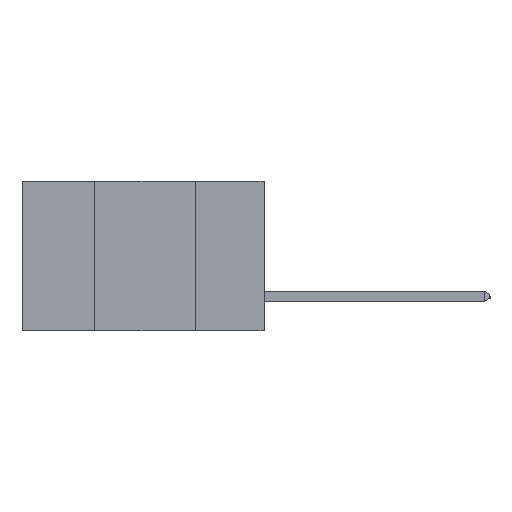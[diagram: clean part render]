
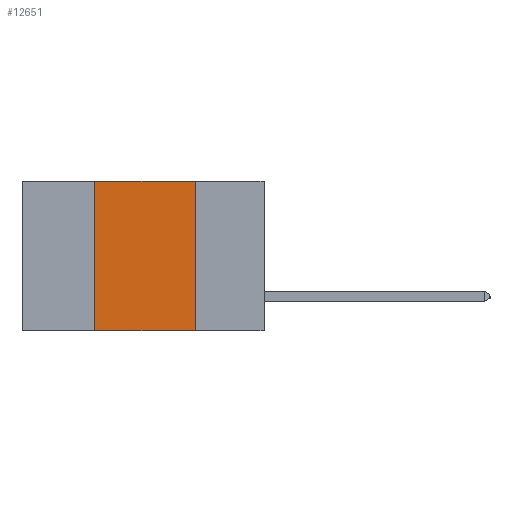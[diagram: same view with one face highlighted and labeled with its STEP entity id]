
A CAD part, left-side view. The second image highlights one B-rep face of the part: STEP entity #12651.
In plain terms, the highlighted planar face has unit normal (-1, 0, 0).
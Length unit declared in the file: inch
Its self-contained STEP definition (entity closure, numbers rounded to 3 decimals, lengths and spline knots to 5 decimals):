
#1932 = DIRECTION ( 'NONE',  ( 0., -1., 0. ) ) ;
#2040 = CARTESIAN_POINT ( 'NONE',  ( 0., 0.17, 0. ) ) ;
#2070 = EDGE_CURVE ( 'NONE', #16121, #6429, #5973, .T. ) ;
#3639 = DIRECTION ( 'NONE',  ( 0., -1., 0. ) ) ;
#4352 = EDGE_CURVE ( 'NONE', #23627, #6429, #24726, .T. ) ;
#4838 = CARTESIAN_POINT ( 'NONE',  ( 0., 0.42, -0.37 ) ) ;
#5973 = LINE ( 'NONE', #14927, #25289 ) ;
#6429 = VERTEX_POINT ( 'NONE', #12253 ) ;
#6909 = LINE ( 'NONE', #28811, #19478 ) ;
#9993 = EDGE_LOOP ( 'NONE', ( #13311, #14872, #23152, #10530 ) ) ;
#10530 = ORIENTED_EDGE ( 'NONE', *, *, #4352, .T. ) ;
#11961 = DIRECTION ( 'NONE',  ( 0., 0., -1. ) ) ;
#12033 = CARTESIAN_POINT ( 'NONE',  ( 0., 0.42, 0. ) ) ;
#12086 = VECTOR ( 'NONE', #1932, 39.37008 ) ;
#12253 = CARTESIAN_POINT ( 'NONE',  ( 0., 0.17, -0.37 ) ) ;
#12651 = ADVANCED_FACE ( 'NONE', ( #31687 ), #29521, .F. ) ;
#13311 = ORIENTED_EDGE ( 'NONE', *, *, #2070, .F. ) ;
#13995 = VERTEX_POINT ( 'NONE', #12033 ) ;
#14640 = CARTESIAN_POINT ( 'NONE',  ( 0., 0.42, 0. ) ) ;
#14872 = ORIENTED_EDGE ( 'NONE', *, *, #27193, .F. ) ;
#14927 = CARTESIAN_POINT ( 'NONE',  ( 0., 0.17, 0. ) ) ;
#16121 = VERTEX_POINT ( 'NONE', #2040 ) ;
#16141 = EDGE_CURVE ( 'NONE', #23627, #13995, #16889, .T. ) ;
#16889 = LINE ( 'NONE', #14640, #20412 ) ;
#16952 = DIRECTION ( 'NONE',  ( 0., 0., -1. ) ) ;
#19478 = VECTOR ( 'NONE', #3639, 39.37008 ) ;
#20412 = VECTOR ( 'NONE', #29733, 39.37008 ) ;
#23152 = ORIENTED_EDGE ( 'NONE', *, *, #16141, .F. ) ;
#23627 = VERTEX_POINT ( 'NONE', #4838 ) ;
#24726 = LINE ( 'NONE', #27666, #12086 ) ;
#25289 = VECTOR ( 'NONE', #11961, 39.37008 ) ;
#27001 = CARTESIAN_POINT ( 'NONE',  ( 0., 0.6, 0. ) ) ;
#27193 = EDGE_CURVE ( 'NONE', #13995, #16121, #6909, .T. ) ;
#27666 = CARTESIAN_POINT ( 'NONE',  ( 0., 0.6, -0.37 ) ) ;
#28166 = AXIS2_PLACEMENT_3D ( 'NONE', #27001, #32050, #16952 ) ;
#28811 = CARTESIAN_POINT ( 'NONE',  ( 0., 0.6, 0. ) ) ;
#29521 = PLANE ( 'NONE',  #28166 ) ;
#29733 = DIRECTION ( 'NONE',  ( 0., 0., 1. ) ) ;
#31687 = FACE_OUTER_BOUND ( 'NONE', #9993, .T. ) ;
#32050 = DIRECTION ( 'NONE',  ( 1., 0., 0. ) ) ;
